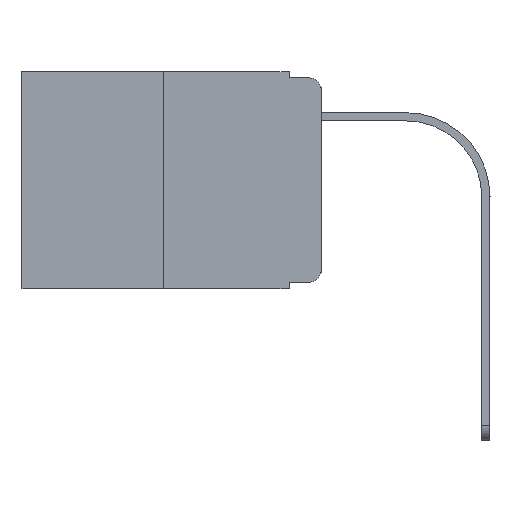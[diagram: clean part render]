
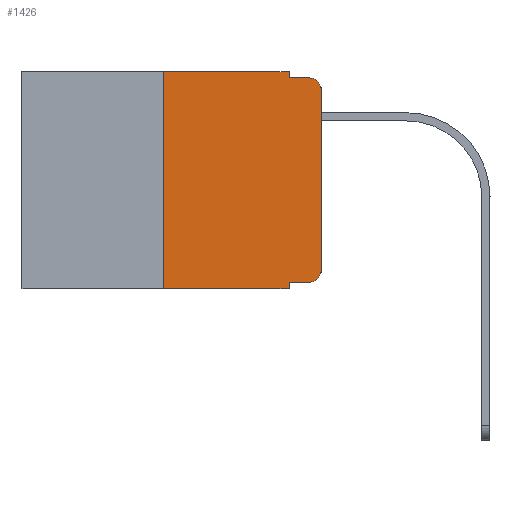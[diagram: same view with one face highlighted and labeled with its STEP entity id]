
A CAD part, left-side view. The second image highlights one B-rep face of the part: STEP entity #1426.
In plain terms, the highlighted planar face has unit normal (-1, 0, 0).
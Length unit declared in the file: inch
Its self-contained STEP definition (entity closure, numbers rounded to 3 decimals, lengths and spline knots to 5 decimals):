
#46 = LINE ( 'NONE', #4446, #13124 ) ;
#58 = EDGE_CURVE ( 'NONE', #5667, #7992, #1835, .T. ) ;
#103 = CARTESIAN_POINT ( 'NONE',  ( 0., 0., -0.03 ) ) ;
#136 = EDGE_CURVE ( 'NONE', #3177, #2163, #12623, .T. ) ;
#194 = CARTESIAN_POINT ( 'NONE',  ( 0., 0.25, 0. ) ) ;
#195 = ORIENTED_EDGE ( 'NONE', *, *, #3592, .F. ) ;
#247 = VECTOR ( 'NONE', #10401, 39.37008 ) ;
#376 = CARTESIAN_POINT ( 'NONE',  ( 0., 0.02, -0.01 ) ) ;
#761 = DIRECTION ( 'NONE',  ( -1., 0., 0. ) ) ;
#1197 = DIRECTION ( 'NONE',  ( 0., 0., -1. ) ) ;
#1426 = ADVANCED_FACE ( 'NONE', ( #3839 ), #11486, .F. ) ;
#1710 = LINE ( 'NONE', #12853, #247 ) ;
#1816 = DIRECTION ( 'NONE',  ( 0., -1., 0. ) ) ;
#1835 = LINE ( 'NONE', #4031, #10341 ) ;
#2026 = VECTOR ( 'NONE', #8620, 39.37008 ) ;
#2039 = DIRECTION ( 'NONE',  ( 0., -1., 0. ) ) ;
#2163 = VERTEX_POINT ( 'NONE', #4793 ) ;
#2180 = ORIENTED_EDGE ( 'NONE', *, *, #58, .T. ) ;
#2274 = VERTEX_POINT ( 'NONE', #376 ) ;
#2593 = ORIENTED_EDGE ( 'NONE', *, *, #8607, .T. ) ;
#2600 = EDGE_CURVE ( 'NONE', #10029, #8363, #4777, .T. ) ;
#2677 = EDGE_CURVE ( 'NONE', #8914, #7992, #1710, .T. ) ;
#2720 = LINE ( 'NONE', #10292, #6720 ) ;
#3177 = VERTEX_POINT ( 'NONE', #11618 ) ;
#3240 = LINE ( 'NONE', #12979, #10671 ) ;
#3592 = EDGE_CURVE ( 'NONE', #8363, #2274, #12600, .T. ) ;
#3623 = AXIS2_PLACEMENT_3D ( 'NONE', #12096, #4331, #1197 ) ;
#3633 = CARTESIAN_POINT ( 'NONE',  ( 0., 0.25, -0.343 ) ) ;
#3839 = FACE_OUTER_BOUND ( 'NONE', #8435, .T. ) ;
#4031 = CARTESIAN_POINT ( 'NONE',  ( 0., 0.473, -0.343 ) ) ;
#4083 = CIRCLE ( 'NONE', #3623, 0.02 ) ;
#4331 = DIRECTION ( 'NONE',  ( -1., 0., 0. ) ) ;
#4385 = DIRECTION ( 'NONE',  ( 0., 0., 1. ) ) ;
#4446 = CARTESIAN_POINT ( 'NONE',  ( 0., 0., 0. ) ) ;
#4452 = DIRECTION ( 'NONE',  ( 0., -1., 0. ) ) ;
#4777 = LINE ( 'NONE', #6895, #6565 ) ;
#4793 = CARTESIAN_POINT ( 'NONE',  ( 0., 0., -0.313 ) ) ;
#5021 = CARTESIAN_POINT ( 'NONE',  ( 0., 0.051, -0.333 ) ) ;
#5099 = DIRECTION ( 'NONE',  ( 0., 0., -1. ) ) ;
#5336 = LINE ( 'NONE', #9692, #2026 ) ;
#5667 = VERTEX_POINT ( 'NONE', #3633 ) ;
#5758 = ORIENTED_EDGE ( 'NONE', *, *, #6412, .T. ) ;
#5937 = CARTESIAN_POINT ( 'NONE',  ( 0., 0.051, -0.01 ) ) ;
#5987 = AXIS2_PLACEMENT_3D ( 'NONE', #8455, #761, #5099 ) ;
#6033 = EDGE_CURVE ( 'NONE', #5667, #8147, #5336, .T. ) ;
#6412 = EDGE_CURVE ( 'NONE', #8518, #2274, #4083, .T. ) ;
#6561 = ORIENTED_EDGE ( 'NONE', *, *, #2677, .F. ) ;
#6565 = VECTOR ( 'NONE', #13631, 39.37008 ) ;
#6720 = VECTOR ( 'NONE', #1816, 39.37008 ) ;
#6736 = CARTESIAN_POINT ( 'NONE',  ( 0., 0.051, -0.01 ) ) ;
#6895 = CARTESIAN_POINT ( 'NONE',  ( 0., 0.051, 0. ) ) ;
#7001 = ORIENTED_EDGE ( 'NONE', *, *, #6033, .F. ) ;
#7054 = EDGE_CURVE ( 'NONE', #8147, #10029, #2720, .T. ) ;
#7136 = CARTESIAN_POINT ( 'NONE',  ( 0., 0.051, -0.343 ) ) ;
#7176 = DIRECTION ( 'NONE',  ( 1., 0., 0. ) ) ;
#7485 = ORIENTED_EDGE ( 'NONE', *, *, #2600, .F. ) ;
#7499 = VECTOR ( 'NONE', #9377, 39.37008 ) ;
#7837 = AXIS2_PLACEMENT_3D ( 'NONE', #11767, #7176, #11556 ) ;
#7992 = VERTEX_POINT ( 'NONE', #7136 ) ;
#8147 = VERTEX_POINT ( 'NONE', #194 ) ;
#8363 = VERTEX_POINT ( 'NONE', #6736 ) ;
#8435 = EDGE_LOOP ( 'NONE', ( #2593, #5758, #195, #7485, #10517, #7001, #2180, #6561, #13066, #12590 ) ) ;
#8455 = CARTESIAN_POINT ( 'NONE',  ( 0., 0.02, -0.313 ) ) ;
#8518 = VERTEX_POINT ( 'NONE', #103 ) ;
#8607 = EDGE_CURVE ( 'NONE', #2163, #8518, #46, .T. ) ;
#8620 = DIRECTION ( 'NONE',  ( 0., 0., 1. ) ) ;
#8914 = VERTEX_POINT ( 'NONE', #5021 ) ;
#9377 = DIRECTION ( 'NONE',  ( 0., -1., 0. ) ) ;
#9692 = CARTESIAN_POINT ( 'NONE',  ( 0., 0.25, 0. ) ) ;
#10029 = VERTEX_POINT ( 'NONE', #11601 ) ;
#10292 = CARTESIAN_POINT ( 'NONE',  ( 0., 0.473, 0. ) ) ;
#10341 = VECTOR ( 'NONE', #2039, 39.37008 ) ;
#10401 = DIRECTION ( 'NONE',  ( 0., 0., -1. ) ) ;
#10517 = ORIENTED_EDGE ( 'NONE', *, *, #7054, .F. ) ;
#10671 = VECTOR ( 'NONE', #4452, 39.37008 ) ;
#11128 = EDGE_CURVE ( 'NONE', #8914, #3177, #3240, .T. ) ;
#11486 = PLANE ( 'NONE',  #7837 ) ;
#11556 = DIRECTION ( 'NONE',  ( 0., 0., -1. ) ) ;
#11601 = CARTESIAN_POINT ( 'NONE',  ( 0., 0.051, 0. ) ) ;
#11618 = CARTESIAN_POINT ( 'NONE',  ( 0., 0.02, -0.333 ) ) ;
#11767 = CARTESIAN_POINT ( 'NONE',  ( 0., 0.473, 0. ) ) ;
#12096 = CARTESIAN_POINT ( 'NONE',  ( 0., 0.02, -0.03 ) ) ;
#12590 = ORIENTED_EDGE ( 'NONE', *, *, #136, .T. ) ;
#12600 = LINE ( 'NONE', #5937, #7499 ) ;
#12623 = CIRCLE ( 'NONE', #5987, 0.02 ) ;
#12853 = CARTESIAN_POINT ( 'NONE',  ( 0., 0.051, 0. ) ) ;
#12979 = CARTESIAN_POINT ( 'NONE',  ( 0., 0.051, -0.333 ) ) ;
#13066 = ORIENTED_EDGE ( 'NONE', *, *, #11128, .T. ) ;
#13124 = VECTOR ( 'NONE', #4385, 39.37008 ) ;
#13631 = DIRECTION ( 'NONE',  ( 0., 0., -1. ) ) ;
